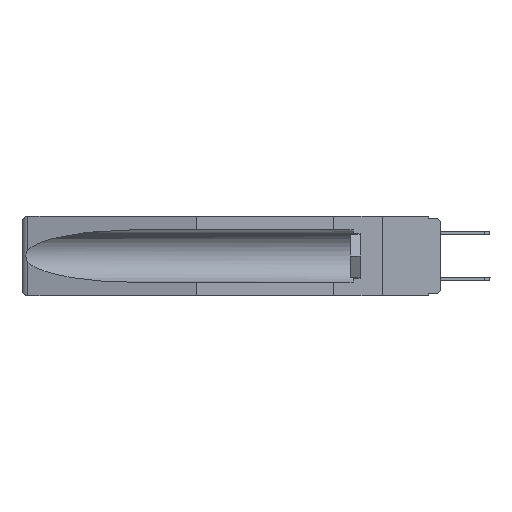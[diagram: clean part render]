
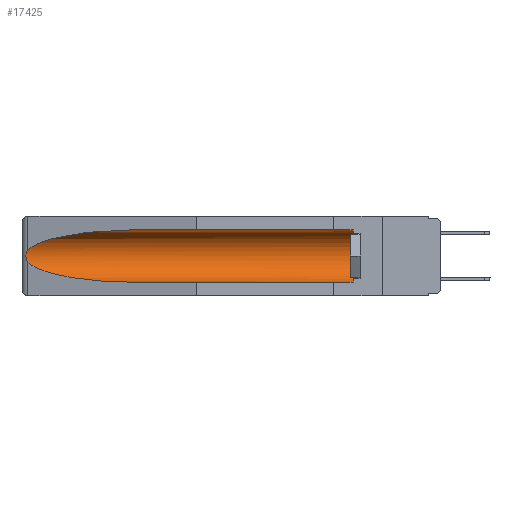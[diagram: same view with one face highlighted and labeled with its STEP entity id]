
A CAD part, left-side view. The second image highlights one B-rep face of the part: STEP entity #17425.
In plain terms, the highlighted cylindrical face has radius 2.857 mm (diameter 5.715 mm), a partial arc.
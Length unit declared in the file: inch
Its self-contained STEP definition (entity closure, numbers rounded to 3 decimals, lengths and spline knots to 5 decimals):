
#53 = CARTESIAN_POINT ( 'NONE',  ( 0.25451, 1.48313, -0.24835 ) ) ;
#343 = DIRECTION ( 'NONE',  ( 0., 1., 0. ) ) ;
#1808 = CARTESIAN_POINT ( 'NONE',  ( 0.2673, 1.5327, -0.16383 ) ) ;
#1963 = VERTEX_POINT ( 'NONE', #9384 ) ;
#2456 = DIRECTION ( 'NONE',  ( 0., 1., 0. ) ) ;
#3190 = CARTESIAN_POINT ( 'NONE',  ( 0.155, 1.07973, -0.284 ) ) ;
#3289 = CIRCLE ( 'NONE', #20311, 0.1125 ) ;
#3654 = DIRECTION ( 'NONE',  ( 0., -1., 0. ) ) ;
#3696 = CARTESIAN_POINT ( 'NONE',  ( 0.2675, 1.53308, -0.17534 ) ) ;
#3818 = CARTESIAN_POINT ( 'NONE',  ( 0.26537, 1.52718, -0.14972 ) ) ;
#3892 = CARTESIAN_POINT ( 'NONE',  ( 0.155, 1.07973, -0.284 ) ) ;
#4068 = VECTOR ( 'NONE', #343, 39.37008 ) ;
#4777 = AXIS2_PLACEMENT_3D ( 'NONE', #25114, #20984, #8971 ) ;
#6424 = CARTESIAN_POINT ( 'NONE',  ( 0.155, -0.30754, -0.284 ) ) ;
#7406 = CARTESIAN_POINT ( 'NONE',  ( 0.155, 0.126, -0.1715 ) ) ;
#7660 = ORIENTED_EDGE ( 'NONE', *, *, #9583, .T. ) ;
#8599 = CARTESIAN_POINT ( 'NONE',  ( 0.155, -0.30754, -0.059 ) ) ;
#8971 = DIRECTION ( 'NONE',  ( 0., 0., 1. ) ) ;
#9074 = CARTESIAN_POINT ( 'NONE',  ( 0.26537, 1.52718, -0.19328 ) ) ;
#9365 = LINE ( 'NONE', #6424, #4068 ) ;
#9384 = CARTESIAN_POINT ( 'NONE',  ( 0.155, 0.126, -0.059 ) ) ;
#9491 = DIRECTION ( 'NONE',  ( 0., 0., 1. ) ) ;
#9583 = EDGE_CURVE ( 'NONE', #13029, #20224, #16251, .T. ) ;
#9665 = EDGE_CURVE ( 'NONE', #23457, #25974, #15153, .T. ) ;
#9698 = B_SPLINE_CURVE_WITH_KNOTS ( 'NONE', 3,
 ( #23806, #11626, #13800, #1808, #15646, #3696, #15811, #17823, #11871, #25901 ),
 .UNSPECIFIED., .F., .F.,
 ( 4, 2, 2, 2, 4 ),
 ( 0., 0.00029, 0.00058, 0.00087, 0.00117 ),
 .UNSPECIFIED. ) ;
#10067 = CARTESIAN_POINT ( 'NONE',  ( 0.21114, 1.30732, -0.284 ) ) ;
#11144 = ORIENTED_EDGE ( 'NONE', *, *, #24166, .T. ) ;
#11507 = CARTESIAN_POINT ( 'NONE',  ( 0.155, 0.126, -0.284 ) ) ;
#11626 = CARTESIAN_POINT ( 'NONE',  ( 0.26597, 1.52961, -0.15275 ) ) ;
#11871 = CARTESIAN_POINT ( 'NONE',  ( 0.26597, 1.5296, -0.19026 ) ) ;
#13029 = VERTEX_POINT ( 'NONE', #9074 ) ;
#13082 = CARTESIAN_POINT ( 'NONE',  ( 0.26537, 1.52718, -0.14972 ) ) ;
#13800 = CARTESIAN_POINT ( 'NONE',  ( 0.26654, 1.53092, -0.15636 ) ) ;
#15054 = EDGE_CURVE ( 'NONE', #25974, #13029, #9698, .T. ) ;
#15153 =( BOUNDED_CURVE ( )  B_SPLINE_CURVE ( 3, ( #23769, #19736, #23852, #3818 ),
 .UNSPECIFIED., .F., .T. ) 
 B_SPLINE_CURVE_WITH_KNOTS ( ( 4, 4 ),
 ( 4.71239, 6.08839 ),
 .UNSPECIFIED. ) 
 CURVE ( )  GEOMETRIC_REPRESENTATION_ITEM ( )  RATIONAL_B_SPLINE_CURVE ( ( 1., 0.848, 0.848, 1. ) ) 
 REPRESENTATION_ITEM ( '' )  );
#15635 = CYLINDRICAL_SURFACE ( 'NONE', #4777, 0.1125 ) ;
#15646 = CARTESIAN_POINT ( 'NONE',  ( 0.2675, 1.53308, -0.16763 ) ) ;
#15811 = CARTESIAN_POINT ( 'NONE',  ( 0.2673, 1.53269, -0.17917 ) ) ;
#15843 = CARTESIAN_POINT ( 'NONE',  ( 0.26537, 1.52718, -0.19328 ) ) ;
#16251 =( BOUNDED_CURVE ( )  B_SPLINE_CURVE ( 3, ( #15843, #53, #10067, #3892 ),
 .UNSPECIFIED., .F., .F. ) 
 B_SPLINE_CURVE_WITH_KNOTS ( ( 4, 4 ),
 ( 0.1948, 1.5708 ),
 .UNSPECIFIED. ) 
 CURVE ( )  GEOMETRIC_REPRESENTATION_ITEM ( )  RATIONAL_B_SPLINE_CURVE ( ( 1., 0.848, 0.848, 1. ) ) 
 REPRESENTATION_ITEM ( '' )  );
#17425 = ADVANCED_FACE ( 'NONE', ( #19715 ), #15635, .F. ) ;
#17594 = EDGE_CURVE ( 'NONE', #25919, #20224, #9365, .T. ) ;
#17639 = ORIENTED_EDGE ( 'NONE', *, *, #17594, .F. ) ;
#17823 = CARTESIAN_POINT ( 'NONE',  ( 0.26655, 1.53094, -0.18657 ) ) ;
#18833 = CARTESIAN_POINT ( 'NONE',  ( 0.155, 1.07973, -0.059 ) ) ;
#19257 = ORIENTED_EDGE ( 'NONE', *, *, #21504, .T. ) ;
#19715 = FACE_OUTER_BOUND ( 'NONE', #25401, .T. ) ;
#19736 = CARTESIAN_POINT ( 'NONE',  ( 0.21114, 1.30732, -0.059 ) ) ;
#20224 = VERTEX_POINT ( 'NONE', #3190 ) ;
#20311 = AXIS2_PLACEMENT_3D ( 'NONE', #7406, #3654, #9491 ) ;
#20984 = DIRECTION ( 'NONE',  ( 0., 1., 0. ) ) ;
#21504 = EDGE_CURVE ( 'NONE', #1963, #23457, #24381, .T. ) ;
#22158 = VECTOR ( 'NONE', #2456, 39.37008 ) ;
#22631 = ORIENTED_EDGE ( 'NONE', *, *, #15054, .T. ) ;
#23457 = VERTEX_POINT ( 'NONE', #18833 ) ;
#23769 = CARTESIAN_POINT ( 'NONE',  ( 0.155, 1.07973, -0.059 ) ) ;
#23806 = CARTESIAN_POINT ( 'NONE',  ( 0.26537, 1.52718, -0.14972 ) ) ;
#23852 = CARTESIAN_POINT ( 'NONE',  ( 0.25451, 1.48313, -0.09465 ) ) ;
#24166 = EDGE_CURVE ( 'NONE', #25919, #1963, #3289, .T. ) ;
#24381 = LINE ( 'NONE', #8599, #22158 ) ;
#25114 = CARTESIAN_POINT ( 'NONE',  ( 0.155, -0.30754, -0.1715 ) ) ;
#25327 = ORIENTED_EDGE ( 'NONE', *, *, #9665, .T. ) ;
#25401 = EDGE_LOOP ( 'NONE', ( #25327, #22631, #7660, #17639, #11144, #19257 ) ) ;
#25901 = CARTESIAN_POINT ( 'NONE',  ( 0.26537, 1.52718, -0.19328 ) ) ;
#25919 = VERTEX_POINT ( 'NONE', #11507 ) ;
#25974 = VERTEX_POINT ( 'NONE', #13082 ) ;
